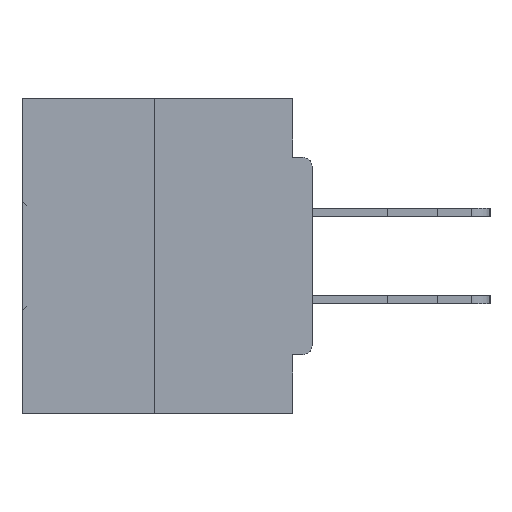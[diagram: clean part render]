
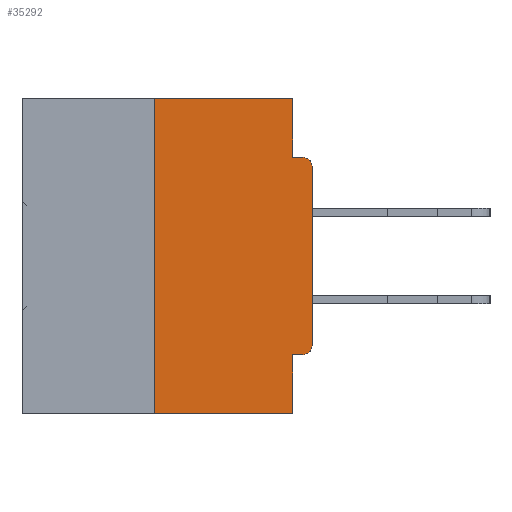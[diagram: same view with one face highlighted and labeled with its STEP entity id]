
A CAD part, left-side view. The second image highlights one B-rep face of the part: STEP entity #35292.
In plain terms, the highlighted planar face has unit normal (-1, 0, 0).
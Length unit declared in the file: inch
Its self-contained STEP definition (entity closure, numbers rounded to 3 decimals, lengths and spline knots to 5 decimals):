
#29 = DIRECTION ( 'NONE',  ( 0., 0., -1. ) ) ;
#667 = EDGE_CURVE ( 'NONE', #8315, #14678, #24075, .T. ) ;
#750 = VERTEX_POINT ( 'NONE', #9962 ) ;
#795 = CARTESIAN_POINT ( 'NONE',  ( 0., 0.46, -0.5 ) ) ;
#2512 = CARTESIAN_POINT ( 'NONE',  ( 0., 0., 0. ) ) ;
#2768 = VERTEX_POINT ( 'NONE', #3566 ) ;
#3507 = CARTESIAN_POINT ( 'NONE',  ( 0., 0.46, 0. ) ) ;
#3566 = CARTESIAN_POINT ( 'NONE',  ( 0., 0.031, -0.5 ) ) ;
#3614 = DIRECTION ( 'NONE',  ( 0., 1., 0. ) ) ;
#4033 = VECTOR ( 'NONE', #38019, 39.37008 ) ;
#5469 = DIRECTION ( 'NONE',  ( 0., 0., 1. ) ) ;
#5690 = EDGE_CURVE ( 'NONE', #19661, #16779, #10555, .T. ) ;
#5692 = CARTESIAN_POINT ( 'NONE',  ( 0., 0.015, -0.1085 ) ) ;
#7391 = CARTESIAN_POINT ( 'NONE',  ( 0., 0.015, -0.4065 ) ) ;
#8054 = DIRECTION ( 'NONE',  ( 0., -1., 0. ) ) ;
#8315 = VERTEX_POINT ( 'NONE', #44027 ) ;
#8541 = ORIENTED_EDGE ( 'NONE', *, *, #20209, .F. ) ;
#9590 = VECTOR ( 'NONE', #8054, 39.37008 ) ;
#9750 = ORIENTED_EDGE ( 'NONE', *, *, #19975, .T. ) ;
#9902 = ORIENTED_EDGE ( 'NONE', *, *, #32336, .T. ) ;
#9962 = CARTESIAN_POINT ( 'NONE',  ( 0., 0.25, 0. ) ) ;
#10210 = CARTESIAN_POINT ( 'NONE',  ( 0., 0., -0.0935 ) ) ;
#10555 = LINE ( 'NONE', #26254, #21235 ) ;
#10918 = ORIENTED_EDGE ( 'NONE', *, *, #41906, .F. ) ;
#12420 = LINE ( 'NONE', #795, #9590 ) ;
#12494 = VERTEX_POINT ( 'NONE', #45225 ) ;
#13986 = DIRECTION ( 'NONE',  ( 0., -1., 0. ) ) ;
#14037 = DIRECTION ( 'NONE',  ( 0., 0., 1. ) ) ;
#14678 = VERTEX_POINT ( 'NONE', #25970 ) ;
#16679 = EDGE_CURVE ( 'NONE', #33330, #2768, #19883, .T. ) ;
#16779 = VERTEX_POINT ( 'NONE', #35768 ) ;
#17699 = LINE ( 'NONE', #44520, #27209 ) ;
#17768 = AXIS2_PLACEMENT_3D ( 'NONE', #3507, #21628, #35907 ) ;
#18286 = VECTOR ( 'NONE', #14037, 39.37008 ) ;
#19159 = DIRECTION ( 'NONE',  ( 0., 0., -1. ) ) ;
#19620 = AXIS2_PLACEMENT_3D ( 'NONE', #24272, #38714, #32102 ) ;
#19661 = VERTEX_POINT ( 'NONE', #29756 ) ;
#19778 = CARTESIAN_POINT ( 'NONE',  ( 0., 0.031, -0.4065 ) ) ;
#19883 = LINE ( 'NONE', #21642, #26667 ) ;
#19975 = EDGE_CURVE ( 'NONE', #41243, #12494, #31087, .T. ) ;
#20209 = EDGE_CURVE ( 'NONE', #750, #19661, #28233, .T. ) ;
#20833 = ORIENTED_EDGE ( 'NONE', *, *, #34419, .F. ) ;
#21185 = VECTOR ( 'NONE', #3614, 39.37008 ) ;
#21235 = VECTOR ( 'NONE', #19159, 39.37008 ) ;
#21628 = DIRECTION ( 'NONE',  ( 1., 0., 0. ) ) ;
#21642 = CARTESIAN_POINT ( 'NONE',  ( 0., 0.031, -0.5 ) ) ;
#24075 = CIRCLE ( 'NONE', #43841, 0.015 ) ;
#24272 = CARTESIAN_POINT ( 'NONE',  ( 0., 0.015, -0.3915 ) ) ;
#25970 = CARTESIAN_POINT ( 'NONE',  ( 0., 0.015, -0.0935 ) ) ;
#26254 = CARTESIAN_POINT ( 'NONE',  ( 0., 0.031, 0. ) ) ;
#26667 = VECTOR ( 'NONE', #29, 39.37008 ) ;
#27209 = VECTOR ( 'NONE', #5469, 39.37008 ) ;
#27472 = CARTESIAN_POINT ( 'NONE',  ( 0., 0., -0.4065 ) ) ;
#28233 = LINE ( 'NONE', #37854, #4033 ) ;
#29318 = EDGE_CURVE ( 'NONE', #33920, #2768, #12420, .T. ) ;
#29756 = CARTESIAN_POINT ( 'NONE',  ( 0., 0.031, 0. ) ) ;
#30712 = EDGE_CURVE ( 'NONE', #16779, #14678, #38132, .T. ) ;
#31087 = CIRCLE ( 'NONE', #19620, 0.015 ) ;
#31797 = EDGE_LOOP ( 'NONE', ( #8541, #20833, #36415, #46594, #10918, #9750, #9902, #36693, #33599, #33782 ) ) ;
#32102 = DIRECTION ( 'NONE',  ( 0., 0., -1. ) ) ;
#32336 = EDGE_CURVE ( 'NONE', #12494, #8315, #35786, .T. ) ;
#32425 = LINE ( 'NONE', #27472, #21185 ) ;
#33330 = VERTEX_POINT ( 'NONE', #19778 ) ;
#33599 = ORIENTED_EDGE ( 'NONE', *, *, #30712, .F. ) ;
#33782 = ORIENTED_EDGE ( 'NONE', *, *, #5690, .F. ) ;
#33920 = VERTEX_POINT ( 'NONE', #44461 ) ;
#34172 = DIRECTION ( 'NONE',  ( -1., 0., 0. ) ) ;
#34419 = EDGE_CURVE ( 'NONE', #33920, #750, #17699, .T. ) ;
#35292 = ADVANCED_FACE ( 'NONE', ( #35585 ), #40002, .F. ) ;
#35585 = FACE_OUTER_BOUND ( 'NONE', #31797, .T. ) ;
#35768 = CARTESIAN_POINT ( 'NONE',  ( 0., 0.031, -0.0935 ) ) ;
#35786 = LINE ( 'NONE', #2512, #18286 ) ;
#35907 = DIRECTION ( 'NONE',  ( 0., 0., -1. ) ) ;
#36415 = ORIENTED_EDGE ( 'NONE', *, *, #29318, .T. ) ;
#36693 = ORIENTED_EDGE ( 'NONE', *, *, #667, .T. ) ;
#37854 = CARTESIAN_POINT ( 'NONE',  ( 0., 0.46, 0. ) ) ;
#38019 = DIRECTION ( 'NONE',  ( 0., -1., 0. ) ) ;
#38132 = LINE ( 'NONE', #10210, #46615 ) ;
#38714 = DIRECTION ( 'NONE',  ( -1., 0., 0. ) ) ;
#40002 = PLANE ( 'NONE',  #17768 ) ;
#41243 = VERTEX_POINT ( 'NONE', #7391 ) ;
#41906 = EDGE_CURVE ( 'NONE', #41243, #33330, #32425, .T. ) ;
#43841 = AXIS2_PLACEMENT_3D ( 'NONE', #5692, #34172, #45533 ) ;
#44027 = CARTESIAN_POINT ( 'NONE',  ( 0., 0., -0.1085 ) ) ;
#44461 = CARTESIAN_POINT ( 'NONE',  ( 0., 0.25, -0.5 ) ) ;
#44520 = CARTESIAN_POINT ( 'NONE',  ( 0., 0.25, 0. ) ) ;
#45225 = CARTESIAN_POINT ( 'NONE',  ( 0., 0., -0.3915 ) ) ;
#45533 = DIRECTION ( 'NONE',  ( 0., 0., -1. ) ) ;
#46594 = ORIENTED_EDGE ( 'NONE', *, *, #16679, .F. ) ;
#46615 = VECTOR ( 'NONE', #13986, 39.37008 ) ;
